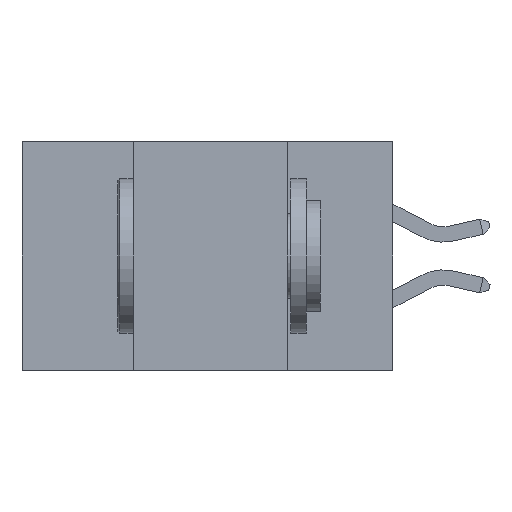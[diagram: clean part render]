
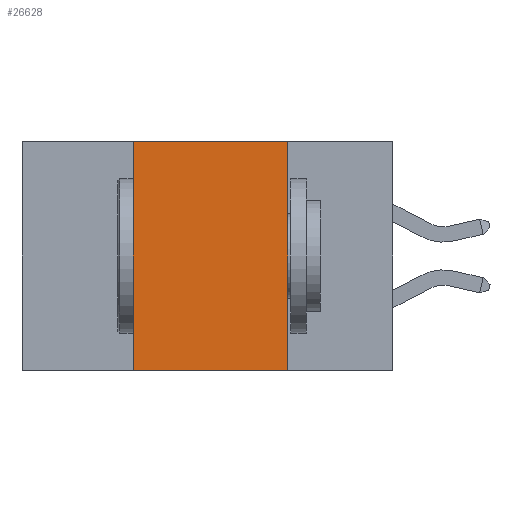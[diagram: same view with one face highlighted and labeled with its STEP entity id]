
A CAD part, left-side view. The second image highlights one B-rep face of the part: STEP entity #26628.
In plain terms, the highlighted planar face has unit normal (-1, 0, 0).
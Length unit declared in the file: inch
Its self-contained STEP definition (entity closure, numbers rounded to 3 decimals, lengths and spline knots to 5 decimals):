
#1784 = DIRECTION ( 'NONE',  ( 0., 0., -1. ) ) ;
#2797 = LINE ( 'NONE', #14109, #20227 ) ;
#2934 = VERTEX_POINT ( 'NONE', #24026 ) ;
#6294 = CARTESIAN_POINT ( 'NONE',  ( 0., 0.6, 0. ) ) ;
#7414 = LINE ( 'NONE', #8000, #12768 ) ;
#8000 = CARTESIAN_POINT ( 'NONE',  ( 0., 0.42, 0. ) ) ;
#8566 = DIRECTION ( 'NONE',  ( 1., 0., 0. ) ) ;
#10581 = ORIENTED_EDGE ( 'NONE', *, *, #12653, .F. ) ;
#11332 = VERTEX_POINT ( 'NONE', #12320 ) ;
#11362 = CARTESIAN_POINT ( 'NONE',  ( 0., 0.42, 0. ) ) ;
#11991 = VECTOR ( 'NONE', #1784, 39.37008 ) ;
#12320 = CARTESIAN_POINT ( 'NONE',  ( 0., 0.17, -0.37 ) ) ;
#12653 = EDGE_CURVE ( 'NONE', #13206, #13142, #22372, .T. ) ;
#12711 = LINE ( 'NONE', #28993, #11991 ) ;
#12768 = VECTOR ( 'NONE', #28439, 39.37008 ) ;
#13142 = VERTEX_POINT ( 'NONE', #20193 ) ;
#13206 = VERTEX_POINT ( 'NONE', #11362 ) ;
#14109 = CARTESIAN_POINT ( 'NONE',  ( 0., 0.6, -0.37 ) ) ;
#15053 = FACE_OUTER_BOUND ( 'NONE', #19142, .T. ) ;
#16407 = DIRECTION ( 'NONE',  ( 0., -1., 0. ) ) ;
#16797 = EDGE_CURVE ( 'NONE', #2934, #11332, #2797, .T. ) ;
#19142 = EDGE_LOOP ( 'NONE', ( #28307, #10581, #21590, #21256 ) ) ;
#19319 = AXIS2_PLACEMENT_3D ( 'NONE', #6294, #8566, #24428 ) ;
#20193 = CARTESIAN_POINT ( 'NONE',  ( 0., 0.17, 0. ) ) ;
#20227 = VECTOR ( 'NONE', #16407, 39.37008 ) ;
#21256 = ORIENTED_EDGE ( 'NONE', *, *, #16797, .T. ) ;
#21590 = ORIENTED_EDGE ( 'NONE', *, *, #23776, .F. ) ;
#22161 = PLANE ( 'NONE',  #19319 ) ;
#22372 = LINE ( 'NONE', #27556, #27686 ) ;
#23087 = DIRECTION ( 'NONE',  ( 0., -1., 0. ) ) ;
#23776 = EDGE_CURVE ( 'NONE', #2934, #13206, #7414, .T. ) ;
#24026 = CARTESIAN_POINT ( 'NONE',  ( 0., 0.42, -0.37 ) ) ;
#24428 = DIRECTION ( 'NONE',  ( 0., 0., -1. ) ) ;
#24701 = EDGE_CURVE ( 'NONE', #13142, #11332, #12711, .T. ) ;
#26628 = ADVANCED_FACE ( 'NONE', ( #15053 ), #22161, .F. ) ;
#27556 = CARTESIAN_POINT ( 'NONE',  ( 0., 0.6, 0. ) ) ;
#27686 = VECTOR ( 'NONE', #23087, 39.37008 ) ;
#28307 = ORIENTED_EDGE ( 'NONE', *, *, #24701, .F. ) ;
#28439 = DIRECTION ( 'NONE',  ( 0., 0., 1. ) ) ;
#28993 = CARTESIAN_POINT ( 'NONE',  ( 0., 0.17, 0. ) ) ;
